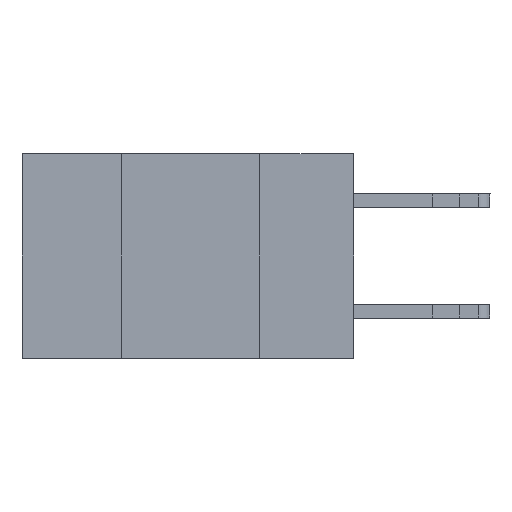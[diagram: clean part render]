
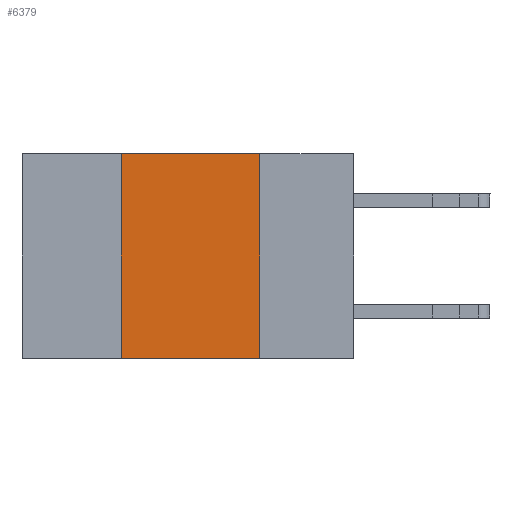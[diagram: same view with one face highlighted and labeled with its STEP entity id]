
A CAD part, left-side view. The second image highlights one B-rep face of the part: STEP entity #6379.
In plain terms, the highlighted planar face has unit normal (-1, 0, 0).
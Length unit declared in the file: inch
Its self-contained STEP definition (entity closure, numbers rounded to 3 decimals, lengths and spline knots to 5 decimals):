
#227 = CARTESIAN_POINT ( 'NONE',  ( 0., 0.17, 0. ) ) ;
#825 = EDGE_CURVE ( 'NONE', #9414, #4548, #15676, .T. ) ;
#1547 = EDGE_CURVE ( 'NONE', #4548, #19091, #13610, .T. ) ;
#2024 = ORIENTED_EDGE ( 'NONE', *, *, #5488, .F. ) ;
#2397 = DIRECTION ( 'NONE',  ( 0., -1., 0. ) ) ;
#2446 = CARTESIAN_POINT ( 'NONE',  ( 0., 0.17, 0. ) ) ;
#3326 = CARTESIAN_POINT ( 'NONE',  ( 0., 0.17, -0.37 ) ) ;
#3713 = LINE ( 'NONE', #15747, #13718 ) ;
#4061 = VECTOR ( 'NONE', #2397, 39.37008 ) ;
#4548 = VERTEX_POINT ( 'NONE', #2446 ) ;
#5251 = EDGE_CURVE ( 'NONE', #10705, #19091, #3713, .T. ) ;
#5488 = EDGE_CURVE ( 'NONE', #10705, #9414, #5940, .T. ) ;
#5940 = LINE ( 'NONE', #17294, #6593 ) ;
#6277 = DIRECTION ( 'NONE',  ( 0., 0., -1. ) ) ;
#6379 = ADVANCED_FACE ( 'NONE', ( #16364 ), #8831, .F. ) ;
#6593 = VECTOR ( 'NONE', #9950, 39.37008 ) ;
#6649 = CARTESIAN_POINT ( 'NONE',  ( 0., 0.42, -0.37 ) ) ;
#8831 = PLANE ( 'NONE',  #17453 ) ;
#8926 = DIRECTION ( 'NONE',  ( 1., 0., 0. ) ) ;
#9057 = DIRECTION ( 'NONE',  ( 0., 0., -1. ) ) ;
#9414 = VERTEX_POINT ( 'NONE', #9850 ) ;
#9784 = CARTESIAN_POINT ( 'NONE',  ( 0., 0.6, 0. ) ) ;
#9850 = CARTESIAN_POINT ( 'NONE',  ( 0., 0.42, 0. ) ) ;
#9950 = DIRECTION ( 'NONE',  ( 0., 0., 1. ) ) ;
#10705 = VERTEX_POINT ( 'NONE', #6649 ) ;
#11009 = DIRECTION ( 'NONE',  ( 0., -1., 0. ) ) ;
#11032 = ORIENTED_EDGE ( 'NONE', *, *, #825, .F. ) ;
#11353 = VECTOR ( 'NONE', #9057, 39.37008 ) ;
#11681 = ORIENTED_EDGE ( 'NONE', *, *, #1547, .F. ) ;
#13610 = LINE ( 'NONE', #227, #11353 ) ;
#13718 = VECTOR ( 'NONE', #11009, 39.37008 ) ;
#13956 = ORIENTED_EDGE ( 'NONE', *, *, #5251, .T. ) ;
#15115 = CARTESIAN_POINT ( 'NONE',  ( 0., 0.6, 0. ) ) ;
#15676 = LINE ( 'NONE', #9784, #4061 ) ;
#15747 = CARTESIAN_POINT ( 'NONE',  ( 0., 0.6, -0.37 ) ) ;
#16364 = FACE_OUTER_BOUND ( 'NONE', #18731, .T. ) ;
#17294 = CARTESIAN_POINT ( 'NONE',  ( 0., 0.42, 0. ) ) ;
#17453 = AXIS2_PLACEMENT_3D ( 'NONE', #15115, #8926, #6277 ) ;
#18731 = EDGE_LOOP ( 'NONE', ( #11681, #11032, #2024, #13956 ) ) ;
#19091 = VERTEX_POINT ( 'NONE', #3326 ) ;
